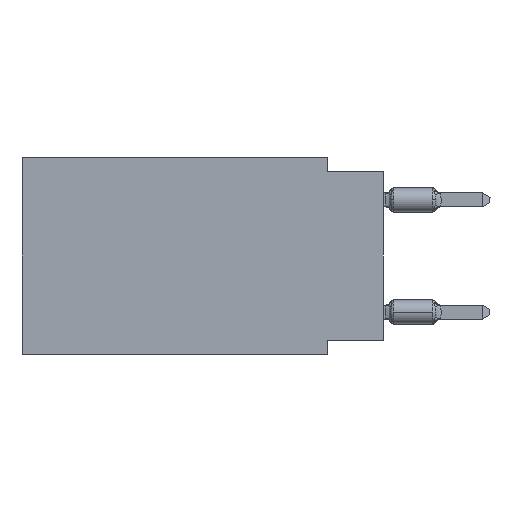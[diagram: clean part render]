
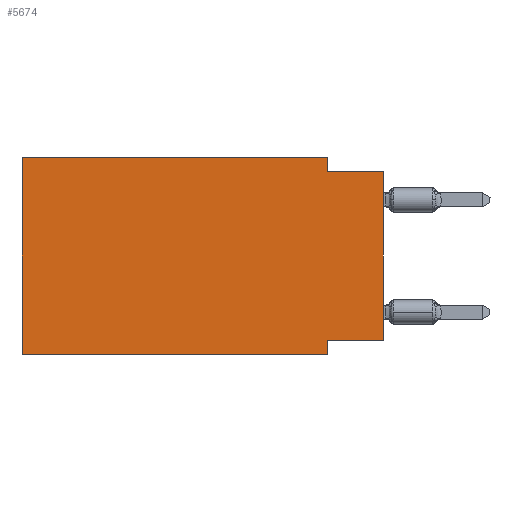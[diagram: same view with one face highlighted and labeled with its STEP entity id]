
A CAD part, left-side view. The second image highlights one B-rep face of the part: STEP entity #5674.
In plain terms, the highlighted planar face has unit normal (-1, 0, 0).
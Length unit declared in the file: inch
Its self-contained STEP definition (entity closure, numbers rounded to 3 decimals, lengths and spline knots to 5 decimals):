
#37 = ORIENTED_EDGE ( 'NONE', *, *, #16302, .F. ) ;
#98 = CARTESIAN_POINT ( 'NONE',  ( 0., 0.1, 0. ) ) ;
#324 = LINE ( 'NONE', #3905, #5741 ) ;
#1164 = EDGE_CURVE ( 'NONE', #13311, #2906, #10773, .T. ) ;
#1222 = FACE_OUTER_BOUND ( 'NONE', #8270, .T. ) ;
#1657 = CARTESIAN_POINT ( 'NONE',  ( 0., 0.1, -0.325 ) ) ;
#2752 = EDGE_CURVE ( 'NONE', #12717, #12000, #4120, .T. ) ;
#2884 = ORIENTED_EDGE ( 'NONE', *, *, #9390, .F. ) ;
#2906 = VERTEX_POINT ( 'NONE', #18551 ) ;
#3593 = DIRECTION ( 'NONE',  ( 0., 0., 1. ) ) ;
#3665 = CARTESIAN_POINT ( 'NONE',  ( 0., 0.645, -0.35 ) ) ;
#3905 = CARTESIAN_POINT ( 'NONE',  ( 0., 0.645, 0. ) ) ;
#4120 = LINE ( 'NONE', #5261, #20150 ) ;
#4437 = CARTESIAN_POINT ( 'NONE',  ( 0., 0., 0. ) ) ;
#4564 = LINE ( 'NONE', #7544, #5757 ) ;
#4912 = DIRECTION ( 'NONE',  ( 0., 0., -1. ) ) ;
#5108 = CARTESIAN_POINT ( 'NONE',  ( 0., 0., -0.325 ) ) ;
#5261 = CARTESIAN_POINT ( 'NONE',  ( 0., 0.1, 0. ) ) ;
#5674 = ADVANCED_FACE ( 'NONE', ( #1222 ), #7591, .F. ) ;
#5741 = VECTOR ( 'NONE', #3593, 39.37008 ) ;
#5757 = VECTOR ( 'NONE', #20039, 39.37008 ) ;
#6256 = LINE ( 'NONE', #17420, #7380 ) ;
#6451 = LINE ( 'NONE', #12685, #17697 ) ;
#7110 = AXIS2_PLACEMENT_3D ( 'NONE', #10365, #18432, #13839 ) ;
#7299 = ORIENTED_EDGE ( 'NONE', *, *, #1164, .T. ) ;
#7380 = VECTOR ( 'NONE', #15987, 39.37008 ) ;
#7544 = CARTESIAN_POINT ( 'NONE',  ( 0., 0.645, 0. ) ) ;
#7591 = PLANE ( 'NONE',  #7110 ) ;
#7953 = VERTEX_POINT ( 'NONE', #17645 ) ;
#8270 = EDGE_LOOP ( 'NONE', ( #7299, #18756, #11874, #17932, #37, #14556, #9207, #2884 ) ) ;
#8321 = EDGE_CURVE ( 'NONE', #8979, #7953, #18631, .T. ) ;
#8979 = VERTEX_POINT ( 'NONE', #1657 ) ;
#9207 = ORIENTED_EDGE ( 'NONE', *, *, #8321, .F. ) ;
#9390 = EDGE_CURVE ( 'NONE', #13311, #8979, #6256, .T. ) ;
#9671 = VERTEX_POINT ( 'NONE', #16663 ) ;
#10365 = CARTESIAN_POINT ( 'NONE',  ( 0., 0.645, 0. ) ) ;
#10509 = CARTESIAN_POINT ( 'NONE',  ( 0., 0.645, 0. ) ) ;
#10773 = LINE ( 'NONE', #4437, #10808 ) ;
#10808 = VECTOR ( 'NONE', #10877, 39.37008 ) ;
#10845 = CARTESIAN_POINT ( 'NONE',  ( 0., 0.1, -0.35 ) ) ;
#10877 = DIRECTION ( 'NONE',  ( 0., 0., 1. ) ) ;
#11488 = DIRECTION ( 'NONE',  ( 0., 0., -1. ) ) ;
#11549 = DIRECTION ( 'NONE',  ( 0., -1., 0. ) ) ;
#11874 = ORIENTED_EDGE ( 'NONE', *, *, #2752, .F. ) ;
#12000 = VERTEX_POINT ( 'NONE', #17301 ) ;
#12685 = CARTESIAN_POINT ( 'NONE',  ( 0., 0., -0.025 ) ) ;
#12717 = VERTEX_POINT ( 'NONE', #98 ) ;
#13112 = EDGE_CURVE ( 'NONE', #12000, #2906, #6451, .T. ) ;
#13311 = VERTEX_POINT ( 'NONE', #5108 ) ;
#13839 = DIRECTION ( 'NONE',  ( 0., 0., -1. ) ) ;
#14556 = ORIENTED_EDGE ( 'NONE', *, *, #16723, .T. ) ;
#15987 = DIRECTION ( 'NONE',  ( 0., 1., 0. ) ) ;
#16231 = VECTOR ( 'NONE', #11549, 39.37008 ) ;
#16302 = EDGE_CURVE ( 'NONE', #9671, #18326, #324, .T. ) ;
#16663 = CARTESIAN_POINT ( 'NONE',  ( 0., 0.645, -0.35 ) ) ;
#16723 = EDGE_CURVE ( 'NONE', #9671, #7953, #17624, .T. ) ;
#17301 = CARTESIAN_POINT ( 'NONE',  ( 0., 0.1, -0.025 ) ) ;
#17420 = CARTESIAN_POINT ( 'NONE',  ( 0., 0., -0.325 ) ) ;
#17624 = LINE ( 'NONE', #3665, #16231 ) ;
#17645 = CARTESIAN_POINT ( 'NONE',  ( 0., 0.1, -0.35 ) ) ;
#17697 = VECTOR ( 'NONE', #18722, 39.37008 ) ;
#17932 = ORIENTED_EDGE ( 'NONE', *, *, #19785, .F. ) ;
#18326 = VERTEX_POINT ( 'NONE', #10509 ) ;
#18432 = DIRECTION ( 'NONE',  ( 1., 0., 0. ) ) ;
#18551 = CARTESIAN_POINT ( 'NONE',  ( 0., 0., -0.025 ) ) ;
#18631 = LINE ( 'NONE', #10845, #19419 ) ;
#18722 = DIRECTION ( 'NONE',  ( 0., -1., 0. ) ) ;
#18756 = ORIENTED_EDGE ( 'NONE', *, *, #13112, .F. ) ;
#19419 = VECTOR ( 'NONE', #4912, 39.37008 ) ;
#19785 = EDGE_CURVE ( 'NONE', #18326, #12717, #4564, .T. ) ;
#20039 = DIRECTION ( 'NONE',  ( 0., -1., 0. ) ) ;
#20150 = VECTOR ( 'NONE', #11488, 39.37008 ) ;
